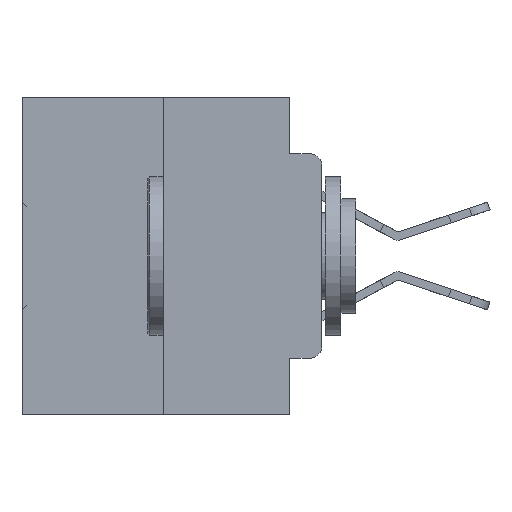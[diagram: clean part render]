
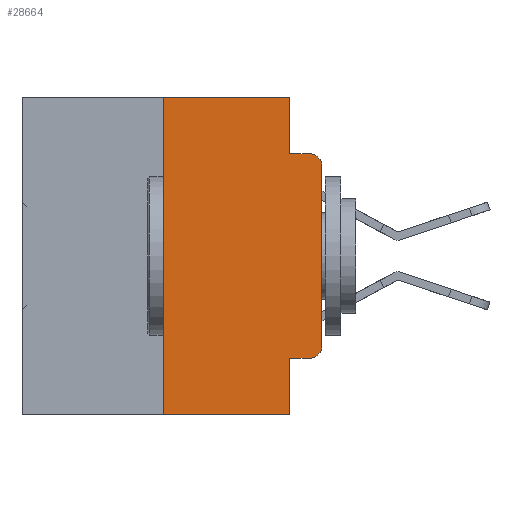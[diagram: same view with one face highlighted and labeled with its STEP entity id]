
A CAD part, left-side view. The second image highlights one B-rep face of the part: STEP entity #28664.
In plain terms, the highlighted planar face has unit normal (-1, 0, 0).
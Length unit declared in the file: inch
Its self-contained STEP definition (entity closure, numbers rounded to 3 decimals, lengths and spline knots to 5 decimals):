
#577 = EDGE_CURVE ( 'NONE', #1567, #20810, #33049, .T. ) ;
#959 = LINE ( 'NONE', #23968, #5837 ) ;
#1567 = VERTEX_POINT ( 'NONE', #28573 ) ;
#1739 = LINE ( 'NONE', #5182, #22084 ) ;
#3308 = DIRECTION ( 'NONE',  ( 0., 0., 1. ) ) ;
#3754 = CARTESIAN_POINT ( 'NONE',  ( 0., 0.051, -0.4115 ) ) ;
#4136 = DIRECTION ( 'NONE',  ( 1., 0., 0. ) ) ;
#4244 = AXIS2_PLACEMENT_3D ( 'NONE', #19766, #8796, #28553 ) ;
#4291 = CARTESIAN_POINT ( 'NONE',  ( 0., 0.051, 0. ) ) ;
#4663 = ORIENTED_EDGE ( 'NONE', *, *, #25219, .F. ) ;
#5010 = DIRECTION ( 'NONE',  ( 0., 0., -1. ) ) ;
#5182 = CARTESIAN_POINT ( 'NONE',  ( 0., 0., 0. ) ) ;
#5633 = DIRECTION ( 'NONE',  ( -1., 0., 0. ) ) ;
#5680 = EDGE_CURVE ( 'NONE', #13209, #10670, #14581, .T. ) ;
#5720 = VECTOR ( 'NONE', #3308, 39.37008 ) ;
#5767 = CARTESIAN_POINT ( 'NONE',  ( 0., 0.473, 0. ) ) ;
#5837 = VECTOR ( 'NONE', #9636, 39.37008 ) ;
#5982 = ORIENTED_EDGE ( 'NONE', *, *, #6586, .F. ) ;
#6036 = ORIENTED_EDGE ( 'NONE', *, *, #26959, .F. ) ;
#6219 = VERTEX_POINT ( 'NONE', #3754 ) ;
#6586 = EDGE_CURVE ( 'NONE', #24753, #25495, #19369, .T. ) ;
#7085 = VECTOR ( 'NONE', #32592, 39.37008 ) ;
#7487 = DIRECTION ( 'NONE',  ( 0., 0., -1. ) ) ;
#8796 = DIRECTION ( 'NONE',  ( -1., 0., 0. ) ) ;
#9110 = CARTESIAN_POINT ( 'NONE',  ( 0., 0.25, 0. ) ) ;
#9636 = DIRECTION ( 'NONE',  ( 0., 0., -1. ) ) ;
#9932 = EDGE_CURVE ( 'NONE', #6219, #34401, #16582, .T. ) ;
#10100 = CARTESIAN_POINT ( 'NONE',  ( 0., 0.25, 0. ) ) ;
#10167 = CARTESIAN_POINT ( 'NONE',  ( 0., 0.051, -0.4115 ) ) ;
#10670 = VERTEX_POINT ( 'NONE', #19032 ) ;
#12027 = CARTESIAN_POINT ( 'NONE',  ( 0., 0.051, -0.5 ) ) ;
#12768 = DIRECTION ( 'NONE',  ( 0., -1., 0. ) ) ;
#13209 = VERTEX_POINT ( 'NONE', #18328 ) ;
#13260 = VERTEX_POINT ( 'NONE', #22260 ) ;
#13591 = CARTESIAN_POINT ( 'NONE',  ( 0., 0., -0.3915 ) ) ;
#13862 = ORIENTED_EDGE ( 'NONE', *, *, #577, .T. ) ;
#14210 = ORIENTED_EDGE ( 'NONE', *, *, #9932, .T. ) ;
#14380 = DIRECTION ( 'NONE',  ( 0., 0., -1. ) ) ;
#14581 = LINE ( 'NONE', #23929, #7085 ) ;
#15674 = VECTOR ( 'NONE', #7487, 39.37008 ) ;
#16095 = ORIENTED_EDGE ( 'NONE', *, *, #16906, .T. ) ;
#16582 = LINE ( 'NONE', #10167, #22758 ) ;
#16767 = VERTEX_POINT ( 'NONE', #13591 ) ;
#16906 = EDGE_CURVE ( 'NONE', #13260, #10670, #19530, .T. ) ;
#17131 = EDGE_CURVE ( 'NONE', #25495, #13209, #959, .T. ) ;
#17335 = CARTESIAN_POINT ( 'NONE',  ( 0., 0.02, -0.3915 ) ) ;
#18067 = CARTESIAN_POINT ( 'NONE',  ( 0., 0.473, 0. ) ) ;
#18328 = CARTESIAN_POINT ( 'NONE',  ( 0., 0.051, -0.0885 ) ) ;
#19032 = CARTESIAN_POINT ( 'NONE',  ( 0., 0.02, -0.0885 ) ) ;
#19369 = LINE ( 'NONE', #5767, #30439 ) ;
#19383 = CARTESIAN_POINT ( 'NONE',  ( 0., 0.473, -0.5 ) ) ;
#19530 = CIRCLE ( 'NONE', #4244, 0.02 ) ;
#19766 = CARTESIAN_POINT ( 'NONE',  ( 0., 0.02, -0.1085 ) ) ;
#19955 = FACE_OUTER_BOUND ( 'NONE', #28372, .T. ) ;
#20258 = LINE ( 'NONE', #9110, #5720 ) ;
#20810 = VERTEX_POINT ( 'NONE', #12027 ) ;
#22084 = VECTOR ( 'NONE', #24915, 39.37008 ) ;
#22260 = CARTESIAN_POINT ( 'NONE',  ( 0., 0., -0.1085 ) ) ;
#22308 = LINE ( 'NONE', #35692, #15674 ) ;
#22758 = VECTOR ( 'NONE', #12768, 39.37008 ) ;
#23929 = CARTESIAN_POINT ( 'NONE',  ( 0., 0.051, -0.0885 ) ) ;
#23968 = CARTESIAN_POINT ( 'NONE',  ( 0., 0.051, 0. ) ) ;
#24524 = AXIS2_PLACEMENT_3D ( 'NONE', #18067, #4136, #5010 ) ;
#24753 = VERTEX_POINT ( 'NONE', #10100 ) ;
#24915 = DIRECTION ( 'NONE',  ( 0., 0., 1. ) ) ;
#25129 = EDGE_CURVE ( 'NONE', #16767, #13260, #1739, .T. ) ;
#25219 = EDGE_CURVE ( 'NONE', #1567, #24753, #20258, .T. ) ;
#25495 = VERTEX_POINT ( 'NONE', #4291 ) ;
#26753 = PLANE ( 'NONE',  #24524 ) ;
#26764 = ORIENTED_EDGE ( 'NONE', *, *, #17131, .F. ) ;
#26959 = EDGE_CURVE ( 'NONE', #6219, #20810, #22308, .T. ) ;
#27194 = ORIENTED_EDGE ( 'NONE', *, *, #5680, .F. ) ;
#28262 = AXIS2_PLACEMENT_3D ( 'NONE', #17335, #5633, #14380 ) ;
#28358 = EDGE_CURVE ( 'NONE', #34401, #16767, #33733, .T. ) ;
#28371 = DIRECTION ( 'NONE',  ( 0., -1., 0. ) ) ;
#28372 = EDGE_LOOP ( 'NONE', ( #32995, #16095, #27194, #26764, #5982, #4663, #13862, #6036, #14210, #31543 ) ) ;
#28553 = DIRECTION ( 'NONE',  ( 0., 0., -1. ) ) ;
#28573 = CARTESIAN_POINT ( 'NONE',  ( 0., 0.25, -0.5 ) ) ;
#28664 = ADVANCED_FACE ( 'NONE', ( #19955 ), #26753, .F. ) ;
#29462 = VECTOR ( 'NONE', #35770, 39.37008 ) ;
#30439 = VECTOR ( 'NONE', #28371, 39.37008 ) ;
#31543 = ORIENTED_EDGE ( 'NONE', *, *, #28358, .T. ) ;
#32592 = DIRECTION ( 'NONE',  ( 0., -1., 0. ) ) ;
#32995 = ORIENTED_EDGE ( 'NONE', *, *, #25129, .T. ) ;
#33049 = LINE ( 'NONE', #19383, #29462 ) ;
#33639 = CARTESIAN_POINT ( 'NONE',  ( 0., 0.02, -0.4115 ) ) ;
#33733 = CIRCLE ( 'NONE', #28262, 0.02 ) ;
#34401 = VERTEX_POINT ( 'NONE', #33639 ) ;
#35692 = CARTESIAN_POINT ( 'NONE',  ( 0., 0.051, 0. ) ) ;
#35770 = DIRECTION ( 'NONE',  ( 0., -1., 0. ) ) ;
